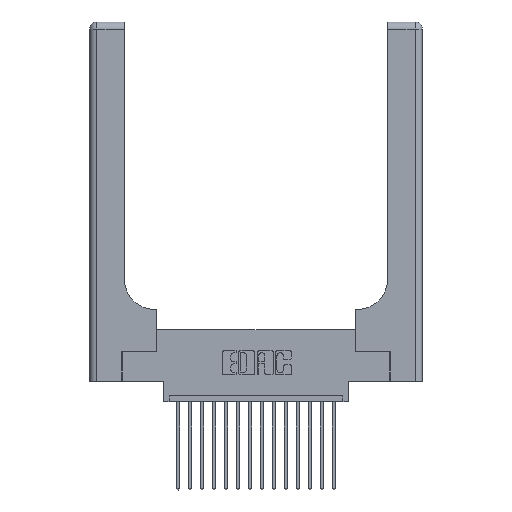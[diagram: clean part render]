
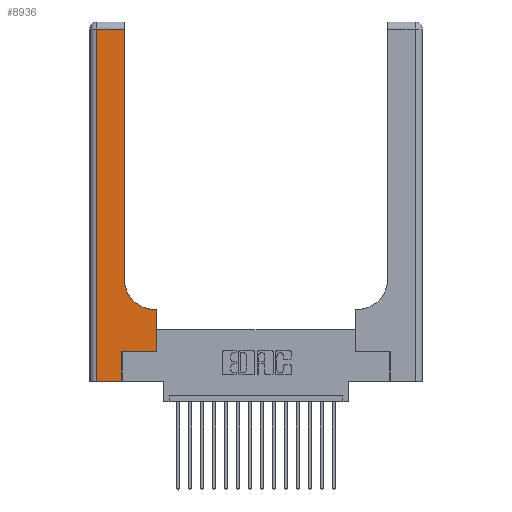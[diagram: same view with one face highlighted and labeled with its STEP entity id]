
A CAD part, top view. The second image highlights one B-rep face of the part: STEP entity #8936.
In plain terms, the highlighted planar face has unit normal (0, 0, 1).
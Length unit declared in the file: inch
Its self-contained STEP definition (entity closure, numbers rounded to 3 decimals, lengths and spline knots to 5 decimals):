
#77 = CARTESIAN_POINT ( 'NONE',  ( 0.2915, 0.85, 0.37 ) ) ;
#724 = VECTOR ( 'NONE', #13072, 39.37008 ) ;
#847 = EDGE_CURVE ( 'NONE', #5259, #13570, #9702, .T. ) ;
#1048 = CARTESIAN_POINT ( 'NONE',  ( 0., 3., 0.37 ) ) ;
#1557 = ORIENTED_EDGE ( 'NONE', *, *, #3763, .T. ) ;
#1713 = CARTESIAN_POINT ( 'NONE',  ( 0.269, 0., 0.37 ) ) ;
#1835 = DIRECTION ( 'NONE',  ( 0., 0., -1. ) ) ;
#2430 = AXIS2_PLACEMENT_3D ( 'NONE', #6112, #1835, #15288 ) ;
#2468 = CARTESIAN_POINT ( 'NONE',  ( 0.5585, 0.25, 0.37 ) ) ;
#2564 = DIRECTION ( 'NONE',  ( -1., 0., 0. ) ) ;
#2585 = ORIENTED_EDGE ( 'NONE', *, *, #6673, .T. ) ;
#2910 = LINE ( 'NONE', #14751, #7885 ) ;
#2940 = LINE ( 'NONE', #15963, #18354 ) ;
#3326 = LINE ( 'NONE', #12886, #18963 ) ;
#3671 = VERTEX_POINT ( 'NONE', #4526 ) ;
#3674 = LINE ( 'NONE', #12191, #6944 ) ;
#3687 = LINE ( 'NONE', #16914, #12471 ) ;
#3763 = EDGE_CURVE ( 'NONE', #17724, #5259, #3687, .T. ) ;
#3825 = CARTESIAN_POINT ( 'NONE',  ( 0.2915, 2.94, 0.37 ) ) ;
#4243 = EDGE_CURVE ( 'NONE', #7070, #3671, #14584, .T. ) ;
#4257 = ORIENTED_EDGE ( 'NONE', *, *, #8076, .T. ) ;
#4495 = DIRECTION ( 'NONE',  ( 0., -1., 0. ) ) ;
#4526 = CARTESIAN_POINT ( 'NONE',  ( 0.06, 2.94, 0.37 ) ) ;
#5259 = VERTEX_POINT ( 'NONE', #18875 ) ;
#5391 = EDGE_CURVE ( 'NONE', #15746, #6458, #2910, .T. ) ;
#5421 = VERTEX_POINT ( 'NONE', #77 ) ;
#5856 = VECTOR ( 'NONE', #18758, 39.37008 ) ;
#6112 = CARTESIAN_POINT ( 'NONE',  ( 0.5415, 0.85, 0.37 ) ) ;
#6208 = FACE_OUTER_BOUND ( 'NONE', #8848, .T. ) ;
#6458 = VERTEX_POINT ( 'NONE', #14035 ) ;
#6479 = VECTOR ( 'NONE', #12492, 39.37008 ) ;
#6673 = EDGE_CURVE ( 'NONE', #13570, #15746, #8775, .T. ) ;
#6944 = VECTOR ( 'NONE', #4495, 39.37008 ) ;
#7019 = CARTESIAN_POINT ( 'NONE',  ( 0.5585, 0.25, 0.37 ) ) ;
#7070 = VERTEX_POINT ( 'NONE', #3825 ) ;
#7214 = ORIENTED_EDGE ( 'NONE', *, *, #4243, .T. ) ;
#7559 = AXIS2_PLACEMENT_3D ( 'NONE', #1048, #11607, #2564 ) ;
#7831 = CARTESIAN_POINT ( 'NONE',  ( 0.269, 0.25, 0.37 ) ) ;
#7885 = VECTOR ( 'NONE', #13227, 39.37008 ) ;
#8076 = EDGE_CURVE ( 'NONE', #3671, #18523, #3674, .T. ) ;
#8414 = DIRECTION ( 'NONE',  ( 0., 1., 0. ) ) ;
#8444 = DIRECTION ( 'NONE',  ( 1., 0., 0. ) ) ;
#8775 = LINE ( 'NONE', #2468, #724 ) ;
#8848 = EDGE_LOOP ( 'NONE', ( #10063, #7214, #4257, #17932, #1557, #15526, #2585, #18141, #9286 ) ) ;
#8899 = CARTESIAN_POINT ( 'NONE',  ( 0.06, 0., 0.37 ) ) ;
#8936 = ADVANCED_FACE ( 'NONE', ( #6208 ), #17658, .F. ) ;
#9286 = ORIENTED_EDGE ( 'NONE', *, *, #14777, .T. ) ;
#9702 = LINE ( 'NONE', #7831, #5856 ) ;
#9736 = EDGE_CURVE ( 'NONE', #5421, #7070, #2940, .T. ) ;
#10063 = ORIENTED_EDGE ( 'NONE', *, *, #9736, .T. ) ;
#10328 = CIRCLE ( 'NONE', #2430, 0.25 ) ;
#10771 = CARTESIAN_POINT ( 'NONE',  ( 0., 2.94, 0.37 ) ) ;
#11563 = EDGE_CURVE ( 'NONE', #18523, #17724, #3326, .T. ) ;
#11607 = DIRECTION ( 'NONE',  ( 0., 0., -1. ) ) ;
#12191 = CARTESIAN_POINT ( 'NONE',  ( 0.06, 3., 0.37 ) ) ;
#12471 = VECTOR ( 'NONE', #15589, 39.37008 ) ;
#12492 = DIRECTION ( 'NONE',  ( -1., 0., 0. ) ) ;
#12835 = CARTESIAN_POINT ( 'NONE',  ( 0.5585, 0.6, 0.37 ) ) ;
#12886 = CARTESIAN_POINT ( 'NONE',  ( 0., 0., 0.37 ) ) ;
#13072 = DIRECTION ( 'NONE',  ( 0., 1., 0. ) ) ;
#13227 = DIRECTION ( 'NONE',  ( -1., 0., 0. ) ) ;
#13570 = VERTEX_POINT ( 'NONE', #7019 ) ;
#14035 = CARTESIAN_POINT ( 'NONE',  ( 0.5415, 0.6, 0.37 ) ) ;
#14584 = LINE ( 'NONE', #10771, #6479 ) ;
#14751 = CARTESIAN_POINT ( 'NONE',  ( 0.2915, 0.6, 0.37 ) ) ;
#14777 = EDGE_CURVE ( 'NONE', #6458, #5421, #10328, .T. ) ;
#15288 = DIRECTION ( 'NONE',  ( 1., 0., 0. ) ) ;
#15526 = ORIENTED_EDGE ( 'NONE', *, *, #847, .T. ) ;
#15589 = DIRECTION ( 'NONE',  ( 0., 1., 0. ) ) ;
#15746 = VERTEX_POINT ( 'NONE', #12835 ) ;
#15963 = CARTESIAN_POINT ( 'NONE',  ( 0.2915, 3., 0.37 ) ) ;
#16914 = CARTESIAN_POINT ( 'NONE',  ( 0.269, 0., 0.37 ) ) ;
#17658 = PLANE ( 'NONE',  #7559 ) ;
#17724 = VERTEX_POINT ( 'NONE', #1713 ) ;
#17932 = ORIENTED_EDGE ( 'NONE', *, *, #11563, .T. ) ;
#18141 = ORIENTED_EDGE ( 'NONE', *, *, #5391, .T. ) ;
#18354 = VECTOR ( 'NONE', #8414, 39.37008 ) ;
#18523 = VERTEX_POINT ( 'NONE', #8899 ) ;
#18758 = DIRECTION ( 'NONE',  ( 1., 0., 0. ) ) ;
#18875 = CARTESIAN_POINT ( 'NONE',  ( 0.269, 0.25, 0.37 ) ) ;
#18963 = VECTOR ( 'NONE', #8444, 39.37008 ) ;
